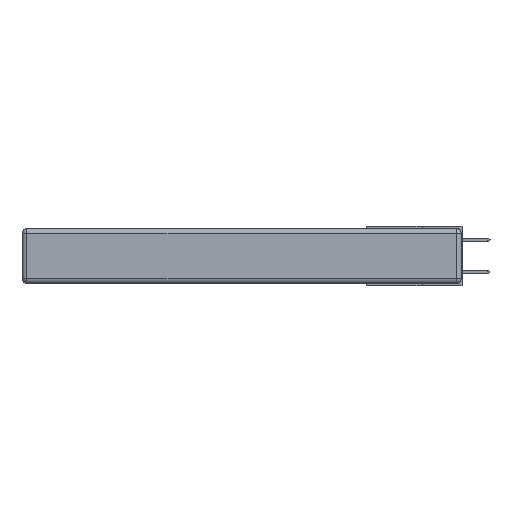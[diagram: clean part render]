
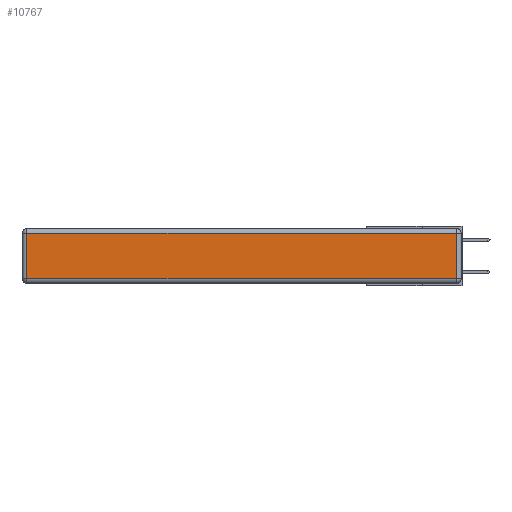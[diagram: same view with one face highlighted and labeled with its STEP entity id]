
A CAD part, left-side view. The second image highlights one B-rep face of the part: STEP entity #10767.
In plain terms, the highlighted planar face has unit normal (-1, 0, 0).
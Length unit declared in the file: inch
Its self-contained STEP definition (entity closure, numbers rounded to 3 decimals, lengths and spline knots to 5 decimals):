
#38 = DIRECTION ( 'NONE',  ( 0., 0., -1. ) ) ;
#489 = ORIENTED_EDGE ( 'NONE', *, *, #28170, .T. ) ;
#881 = VERTEX_POINT ( 'NONE', #19731 ) ;
#940 = ORIENTED_EDGE ( 'NONE', *, *, #17524, .T. ) ;
#3203 = DIRECTION ( 'NONE',  ( 0., 0., 1. ) ) ;
#3290 = PLANE ( 'NONE',  #5674 ) ;
#3370 = EDGE_CURVE ( 'NONE', #30190, #33404, #11247, .T. ) ;
#3791 = LINE ( 'NONE', #8756, #15358 ) ;
#5674 = AXIS2_PLACEMENT_3D ( 'NONE', #26923, #21526, #32103 ) ;
#7102 = CARTESIAN_POINT ( 'NONE',  ( 0., 2.72, -0.03 ) ) ;
#8756 = CARTESIAN_POINT ( 'NONE',  ( 0., 0., -0.313 ) ) ;
#9308 = FACE_OUTER_BOUND ( 'NONE', #15739, .T. ) ;
#9624 = CARTESIAN_POINT ( 'NONE',  ( 0., 2.75, -0.03 ) ) ;
#10767 = ADVANCED_FACE ( 'NONE', ( #9308 ), #3290, .T. ) ;
#11247 = LINE ( 'NONE', #9624, #17426 ) ;
#13727 = LINE ( 'NONE', #31040, #19914 ) ;
#14608 = VECTOR ( 'NONE', #3203, 39.37008 ) ;
#14930 = DIRECTION ( 'NONE',  ( 0., 1., 0. ) ) ;
#15358 = VECTOR ( 'NONE', #19601, 39.37008 ) ;
#15739 = EDGE_LOOP ( 'NONE', ( #22564, #489, #32901, #940 ) ) ;
#16445 = CARTESIAN_POINT ( 'NONE',  ( 0., 0.03, -0.03 ) ) ;
#17426 = VECTOR ( 'NONE', #14930, 39.37008 ) ;
#17524 = EDGE_CURVE ( 'NONE', #33404, #881, #13727, .T. ) ;
#17929 = EDGE_CURVE ( 'NONE', #881, #20022, #3791, .T. ) ;
#19522 = LINE ( 'NONE', #27276, #14608 ) ;
#19601 = DIRECTION ( 'NONE',  ( 0., -1., 0. ) ) ;
#19731 = CARTESIAN_POINT ( 'NONE',  ( 0., 2.72, -0.313 ) ) ;
#19914 = VECTOR ( 'NONE', #38, 39.37008 ) ;
#20022 = VERTEX_POINT ( 'NONE', #26256 ) ;
#21526 = DIRECTION ( 'NONE',  ( -1., 0., 0. ) ) ;
#22564 = ORIENTED_EDGE ( 'NONE', *, *, #17929, .T. ) ;
#26256 = CARTESIAN_POINT ( 'NONE',  ( 0., 0.03, -0.313 ) ) ;
#26923 = CARTESIAN_POINT ( 'NONE',  ( 0., 0., -0.343 ) ) ;
#27276 = CARTESIAN_POINT ( 'NONE',  ( 0., 0.03, -0.343 ) ) ;
#28170 = EDGE_CURVE ( 'NONE', #20022, #30190, #19522, .T. ) ;
#30190 = VERTEX_POINT ( 'NONE', #16445 ) ;
#31040 = CARTESIAN_POINT ( 'NONE',  ( 0., 2.72, -0.343 ) ) ;
#32103 = DIRECTION ( 'NONE',  ( 0., 0., 1. ) ) ;
#32901 = ORIENTED_EDGE ( 'NONE', *, *, #3370, .T. ) ;
#33404 = VERTEX_POINT ( 'NONE', #7102 ) ;
